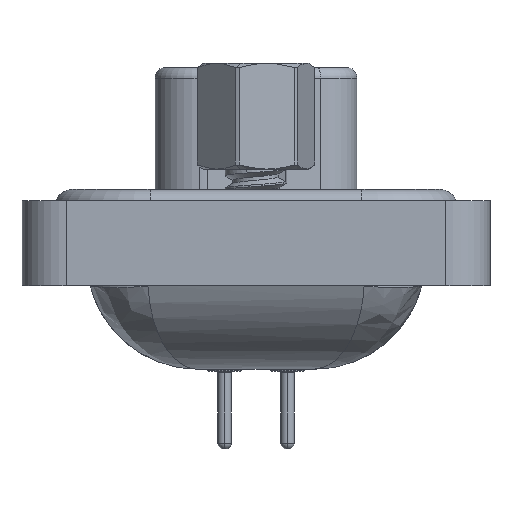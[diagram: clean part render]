
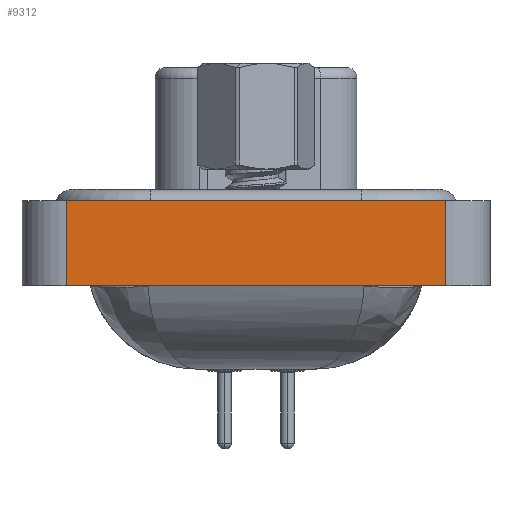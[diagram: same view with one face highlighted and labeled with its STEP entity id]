
A CAD part, left-side view. The second image highlights one B-rep face of the part: STEP entity #9312.
In plain terms, the highlighted planar face has unit normal (-1, 0, 0).
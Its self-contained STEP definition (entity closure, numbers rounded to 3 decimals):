
#168 = EDGE_LOOP ( 'NONE', ( #1209, #3870, #2594, #17929 ) ) ;
#1103 = CARTESIAN_POINT ( 'NONE',  ( -7.35, 8.55, 0.5 ) ) ;
#1209 = ORIENTED_EDGE ( 'NONE', *, *, #8288, .T. ) ;
#1331 = DIRECTION ( 'NONE',  ( 0., -1., 0. ) ) ;
#2070 = VECTOR ( 'NONE', #2674, 1000. ) ;
#2594 = ORIENTED_EDGE ( 'NONE', *, *, #11650, .F. ) ;
#2674 = DIRECTION ( 'NONE',  ( 0., -1., 0. ) ) ;
#2685 = PLANE ( 'NONE',  #17792 ) ;
#3568 = CARTESIAN_POINT ( 'NONE',  ( -7.35, 8.55, -3.35 ) ) ;
#3870 = ORIENTED_EDGE ( 'NONE', *, *, #14177, .F. ) ;
#4473 = VERTEX_POINT ( 'NONE', #3568 ) ;
#4978 = LINE ( 'NONE', #10437, #22717 ) ;
#5363 = LINE ( 'NONE', #12587, #17389 ) ;
#6573 = DIRECTION ( 'NONE',  ( 0., 0., 1. ) ) ;
#8171 = VERTEX_POINT ( 'NONE', #15913 ) ;
#8288 = EDGE_CURVE ( 'NONE', #9192, #8171, #5363, .T. ) ;
#9192 = VERTEX_POINT ( 'NONE', #10853 ) ;
#9312 = ADVANCED_FACE ( 'NONE', ( #15448 ), #2685, .T. ) ;
#10437 = CARTESIAN_POINT ( 'NONE',  ( -7.35, -8.55, 0.5 ) ) ;
#10853 = CARTESIAN_POINT ( 'NONE',  ( -7.35, -8.55, -3.35 ) ) ;
#11650 = EDGE_CURVE ( 'NONE', #4473, #12194, #17437, .T. ) ;
#12194 = VERTEX_POINT ( 'NONE', #1103 ) ;
#12570 = VECTOR ( 'NONE', #15324, 1000. ) ;
#12587 = CARTESIAN_POINT ( 'NONE',  ( -7.35, -8.55, -3.35 ) ) ;
#12709 = DIRECTION ( 'NONE',  ( 0., 0., 1. ) ) ;
#13555 = DIRECTION ( 'NONE',  ( -1., 0., 0. ) ) ;
#14177 = EDGE_CURVE ( 'NONE', #12194, #8171, #4978, .T. ) ;
#15324 = DIRECTION ( 'NONE',  ( 0., 0., 1. ) ) ;
#15448 = FACE_OUTER_BOUND ( 'NONE', #168, .T. ) ;
#15913 = CARTESIAN_POINT ( 'NONE',  ( -7.35, -8.55, 0.5 ) ) ;
#17088 = CARTESIAN_POINT ( 'NONE',  ( -7.35, 8.55, -3.35 ) ) ;
#17090 = CARTESIAN_POINT ( 'NONE',  ( -7.35, -8.55, -3.35 ) ) ;
#17217 = CARTESIAN_POINT ( 'NONE',  ( -7.35, -8.55, -3.35 ) ) ;
#17389 = VECTOR ( 'NONE', #12709, 1000. ) ;
#17437 = LINE ( 'NONE', #17088, #12570 ) ;
#17792 = AXIS2_PLACEMENT_3D ( 'NONE', #17217, #13555, #6573 ) ;
#17929 = ORIENTED_EDGE ( 'NONE', *, *, #18851, .T. ) ;
#18851 = EDGE_CURVE ( 'NONE', #4473, #9192, #22493, .T. ) ;
#22493 = LINE ( 'NONE', #17090, #2070 ) ;
#22717 = VECTOR ( 'NONE', #1331, 1000. ) ;
